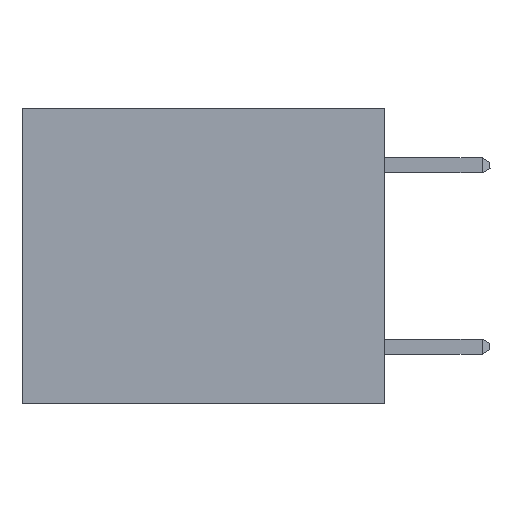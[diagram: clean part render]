
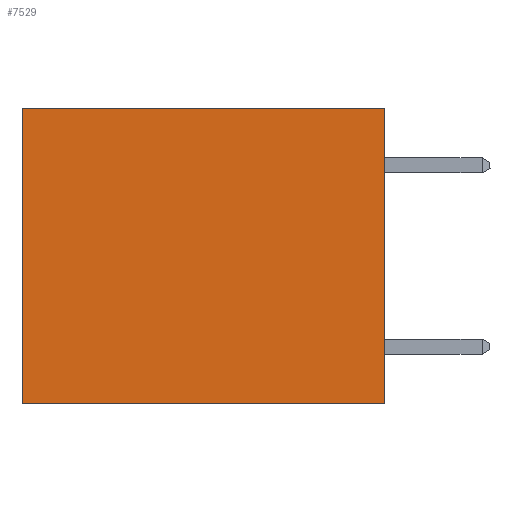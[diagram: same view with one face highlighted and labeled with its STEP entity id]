
A CAD part, left-side view. The second image highlights one B-rep face of the part: STEP entity #7529.
In plain terms, the highlighted planar face has unit normal (-1, 0, 0).
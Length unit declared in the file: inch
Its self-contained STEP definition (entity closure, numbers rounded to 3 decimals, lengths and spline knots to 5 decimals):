
#328 = DIRECTION ( 'NONE',  ( 0., 1., 0. ) ) ;
#335 = ORIENTED_EDGE ( 'NONE', *, *, #20028, .T. ) ;
#346 = LINE ( 'NONE', #1627, #11184 ) ;
#949 = DIRECTION ( 'NONE',  ( 0., 0., -1. ) ) ;
#1627 = CARTESIAN_POINT ( 'NONE',  ( 0.3165, 0., -0.49 ) ) ;
#1758 = DIRECTION ( 'NONE',  ( 0., 0., -1. ) ) ;
#2060 = ORIENTED_EDGE ( 'NONE', *, *, #15263, .F. ) ;
#3308 = LINE ( 'NONE', #15271, #3631 ) ;
#3631 = VECTOR ( 'NONE', #328, 39.37008 ) ;
#4264 = AXIS2_PLACEMENT_3D ( 'NONE', #10201, #5988, #1758 ) ;
#4812 = CARTESIAN_POINT ( 'NONE',  ( 0.3165, 0.6, -0.49 ) ) ;
#5322 = CARTESIAN_POINT ( 'NONE',  ( 0.3165, 0., -0.49 ) ) ;
#5988 = DIRECTION ( 'NONE',  ( 1., 0., 0. ) ) ;
#6518 = VERTEX_POINT ( 'NONE', #20653 ) ;
#6958 = LINE ( 'NONE', #7421, #10882 ) ;
#7421 = CARTESIAN_POINT ( 'NONE',  ( 0.3165, 0.6, -0.49 ) ) ;
#7529 = ADVANCED_FACE ( 'NONE', ( #24797 ), #16431, .F. ) ;
#7620 = VERTEX_POINT ( 'NONE', #5322 ) ;
#8329 = CARTESIAN_POINT ( 'NONE',  ( 0.3165, 0., 0. ) ) ;
#8929 = LINE ( 'NONE', #20511, #18830 ) ;
#10201 = CARTESIAN_POINT ( 'NONE',  ( 0.3165, 0., -0.49 ) ) ;
#10882 = VECTOR ( 'NONE', #949, 39.37008 ) ;
#11173 = EDGE_LOOP ( 'NONE', ( #335, #22906, #2060, #22723 ) ) ;
#11184 = VECTOR ( 'NONE', #16401, 39.37008 ) ;
#15263 = EDGE_CURVE ( 'NONE', #24446, #7620, #346, .T. ) ;
#15271 = CARTESIAN_POINT ( 'NONE',  ( 0.3165, 0., 0. ) ) ;
#15329 = DIRECTION ( 'NONE',  ( 0., 1., 0. ) ) ;
#15901 = EDGE_CURVE ( 'NONE', #24446, #6518, #3308, .T. ) ;
#16401 = DIRECTION ( 'NONE',  ( 0., 0., -1. ) ) ;
#16431 = PLANE ( 'NONE',  #4264 ) ;
#18830 = VECTOR ( 'NONE', #15329, 39.37008 ) ;
#20028 = EDGE_CURVE ( 'NONE', #6518, #22810, #6958, .T. ) ;
#20511 = CARTESIAN_POINT ( 'NONE',  ( 0.3165, 0., -0.49 ) ) ;
#20653 = CARTESIAN_POINT ( 'NONE',  ( 0.3165, 0.6, 0. ) ) ;
#22723 = ORIENTED_EDGE ( 'NONE', *, *, #15901, .T. ) ;
#22810 = VERTEX_POINT ( 'NONE', #4812 ) ;
#22906 = ORIENTED_EDGE ( 'NONE', *, *, #25684, .F. ) ;
#24446 = VERTEX_POINT ( 'NONE', #8329 ) ;
#24797 = FACE_OUTER_BOUND ( 'NONE', #11173, .T. ) ;
#25684 = EDGE_CURVE ( 'NONE', #7620, #22810, #8929, .T. ) ;
